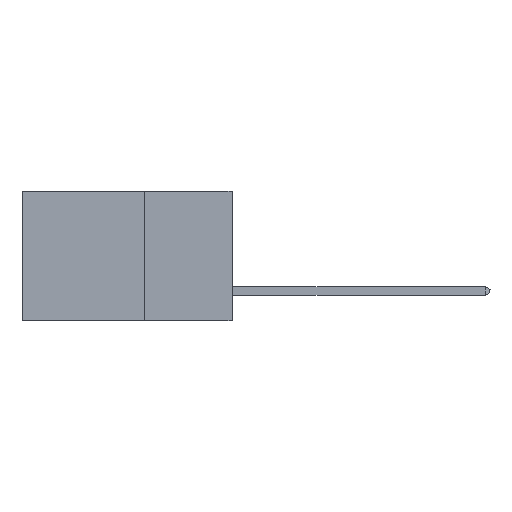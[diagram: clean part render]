
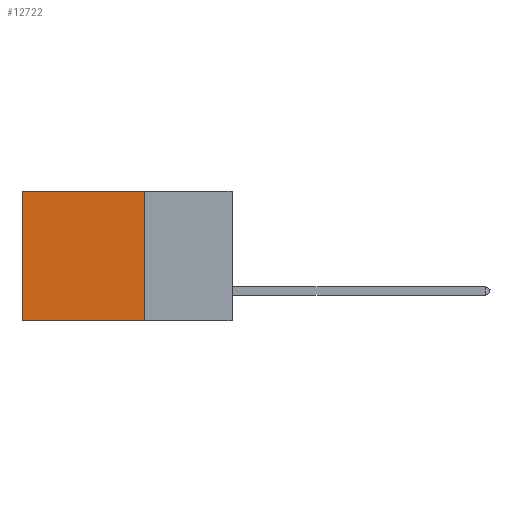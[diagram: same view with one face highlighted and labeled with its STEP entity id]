
A CAD part, left-side view. The second image highlights one B-rep face of the part: STEP entity #12722.
In plain terms, the highlighted planar face has unit normal (-1, 0, 0).
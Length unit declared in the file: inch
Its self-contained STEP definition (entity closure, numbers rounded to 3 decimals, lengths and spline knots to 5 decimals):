
#1751 = AXIS2_PLACEMENT_3D ( 'NONE', #8239, #14258, #5156 ) ;
#1863 = CARTESIAN_POINT ( 'NONE',  ( 0.2875, 0.25, 0. ) ) ;
#2248 = ORIENTED_EDGE ( 'NONE', *, *, #4206, .F. ) ;
#2713 = DIRECTION ( 'NONE',  ( 0., 0., -1. ) ) ;
#3662 = CARTESIAN_POINT ( 'NONE',  ( 0.2875, 0.25, -0.37 ) ) ;
#3825 = VECTOR ( 'NONE', #12242, 39.37008 ) ;
#4206 = EDGE_CURVE ( 'NONE', #10186, #12826, #8291, .T. ) ;
#4874 = DIRECTION ( 'NONE',  ( 0., 1., 0. ) ) ;
#5156 = DIRECTION ( 'NONE',  ( 0., 0., -1. ) ) ;
#5297 = EDGE_LOOP ( 'NONE', ( #14035, #2248, #7688, #14118 ) ) ;
#6052 = CARTESIAN_POINT ( 'NONE',  ( 0.2875, 0.25, 0. ) ) ;
#6662 = FACE_OUTER_BOUND ( 'NONE', #5297, .T. ) ;
#6988 = VECTOR ( 'NONE', #4874, 39.37008 ) ;
#7105 = LINE ( 'NONE', #7140, #12922 ) ;
#7140 = CARTESIAN_POINT ( 'NONE',  ( 0.2875, 0.6, 0. ) ) ;
#7391 = DIRECTION ( 'NONE',  ( 0., 1., 0. ) ) ;
#7688 = ORIENTED_EDGE ( 'NONE', *, *, #13955, .F. ) ;
#7904 = EDGE_CURVE ( 'NONE', #16659, #14819, #10476, .T. ) ;
#8239 = CARTESIAN_POINT ( 'NONE',  ( 0.2875, 0.25, 0. ) ) ;
#8291 = LINE ( 'NONE', #13414, #16861 ) ;
#9172 = CARTESIAN_POINT ( 'NONE',  ( 0.2875, 0.25, 0. ) ) ;
#10186 = VERTEX_POINT ( 'NONE', #3662 ) ;
#10476 = LINE ( 'NONE', #6052, #6988 ) ;
#11106 = EDGE_CURVE ( 'NONE', #14819, #12826, #7105, .T. ) ;
#12242 = DIRECTION ( 'NONE',  ( 0., 0., -1. ) ) ;
#12646 = PLANE ( 'NONE',  #1751 ) ;
#12722 = ADVANCED_FACE ( 'NONE', ( #6662 ), #12646, .F. ) ;
#12826 = VERTEX_POINT ( 'NONE', #14948 ) ;
#12922 = VECTOR ( 'NONE', #2713, 39.37008 ) ;
#13414 = CARTESIAN_POINT ( 'NONE',  ( 0.2875, 0.25, -0.37 ) ) ;
#13955 = EDGE_CURVE ( 'NONE', #16659, #10186, #14285, .T. ) ;
#14035 = ORIENTED_EDGE ( 'NONE', *, *, #11106, .T. ) ;
#14118 = ORIENTED_EDGE ( 'NONE', *, *, #7904, .T. ) ;
#14258 = DIRECTION ( 'NONE',  ( 1., 0., 0. ) ) ;
#14285 = LINE ( 'NONE', #1863, #3825 ) ;
#14819 = VERTEX_POINT ( 'NONE', #16171 ) ;
#14948 = CARTESIAN_POINT ( 'NONE',  ( 0.2875, 0.6, -0.37 ) ) ;
#16171 = CARTESIAN_POINT ( 'NONE',  ( 0.2875, 0.6, 0. ) ) ;
#16659 = VERTEX_POINT ( 'NONE', #9172 ) ;
#16861 = VECTOR ( 'NONE', #7391, 39.37008 ) ;
